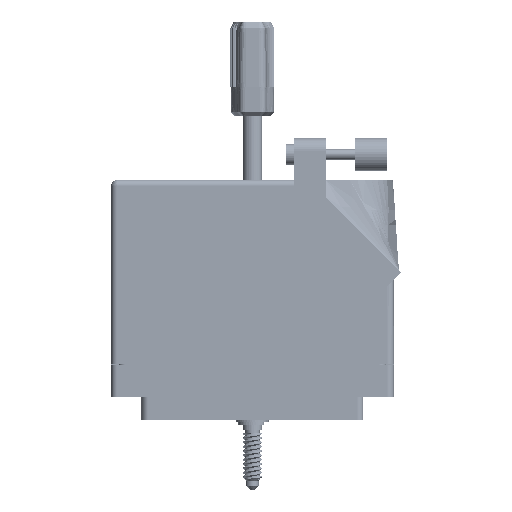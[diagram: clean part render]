
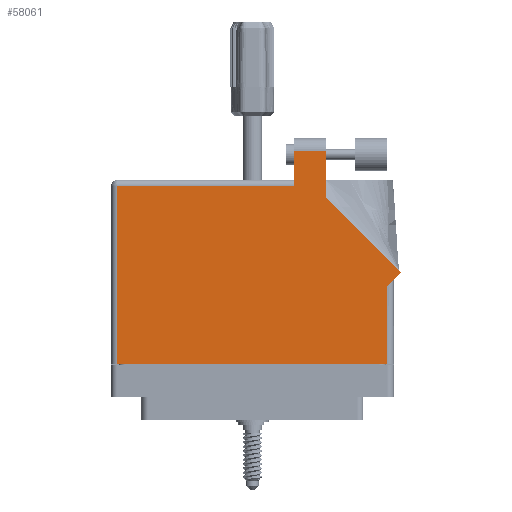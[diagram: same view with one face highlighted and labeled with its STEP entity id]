
A CAD part, front view. The second image highlights one B-rep face of the part: STEP entity #58061.
In plain terms, the highlighted face is planar.
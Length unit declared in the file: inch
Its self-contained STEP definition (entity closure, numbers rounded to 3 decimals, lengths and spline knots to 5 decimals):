
#2322 = VERTEX_POINT ( 'NONE', #53508 ) ;
#4715 = LINE ( 'NONE', #34771, #56115 ) ;
#6312 = DIRECTION ( 'NONE',  ( 0., -1., 0. ) ) ;
#9422 = CARTESIAN_POINT ( 'NONE',  ( 1.297, 0.653, 0.617 ) ) ;
#10979 = VECTOR ( 'NONE', #77867, 39.37008 ) ;
#12098 = AXIS2_PLACEMENT_3D ( 'NONE', #58994, #39095, #46079 ) ;
#12374 = EDGE_CURVE ( 'NONE', #52562, #39592, #4715, .T. ) ;
#12663 = PLANE ( 'NONE',  #12098 ) ;
#14549 = VERTEX_POINT ( 'NONE', #64242 ) ;
#15652 = EDGE_LOOP ( 'NONE', ( #80241, #50006, #67165, #20343, #57111, #83037, #20977, #72256, #41765 ) ) ;
#16289 = CARTESIAN_POINT ( 'NONE',  ( -1.297, -0.1, 0.617 ) ) ;
#16480 = DIRECTION ( 'NONE',  ( 0., 1., 0. ) ) ;
#18268 = CARTESIAN_POINT ( 'NONE',  ( 0.399, 1.613, 0.617 ) ) ;
#18974 = VERTEX_POINT ( 'NONE', #31408 ) ;
#20343 = ORIENTED_EDGE ( 'NONE', *, *, #22584, .T. ) ;
#20977 = ORIENTED_EDGE ( 'NONE', *, *, #83880, .T. ) ;
#22584 = EDGE_CURVE ( 'NONE', #84639, #2322, #63732, .T. ) ;
#23260 = LINE ( 'NONE', #41619, #76675 ) ;
#24016 = CARTESIAN_POINT ( 'NONE',  ( 0.399, 1.675, 0.617 ) ) ;
#26100 = CARTESIAN_POINT ( 'NONE',  ( -1.297, -0.1, 0.617 ) ) ;
#29074 = DIRECTION ( 'NONE',  ( 0., 1., 0. ) ) ;
#30995 = CARTESIAN_POINT ( 'NONE',  ( 1.359, 0.715, 0.617 ) ) ;
#31408 = CARTESIAN_POINT ( 'NONE',  ( 0.399, 1.95, 0.617 ) ) ;
#33461 = EDGE_CURVE ( 'NONE', #49750, #46860, #74212, .T. ) ;
#33723 = EDGE_CURVE ( 'NONE', #14549, #49750, #42667, .T. ) ;
#34771 = CARTESIAN_POINT ( 'NONE',  ( -1.359, -0.1, 0.617 ) ) ;
#36642 = VERTEX_POINT ( 'NONE', #9422 ) ;
#38726 = CARTESIAN_POINT ( 'NONE',  ( 1.42971, 0.78571, 0.617 ) ) ;
#39095 = DIRECTION ( 'NONE',  ( 0., 0., -1. ) ) ;
#39592 = VERTEX_POINT ( 'NONE', #65286 ) ;
#40361 = FACE_OUTER_BOUND ( 'NONE', #15652, .T. ) ;
#41442 = LINE ( 'NONE', #30995, #10979 ) ;
#41619 = CARTESIAN_POINT ( 'NONE',  ( 0.399, 1.95, 0.617 ) ) ;
#41765 = ORIENTED_EDGE ( 'NONE', *, *, #33723, .T. ) ;
#42085 = LINE ( 'NONE', #24016, #53551 ) ;
#42655 = VECTOR ( 'NONE', #29074, 39.37008 ) ;
#42667 = LINE ( 'NONE', #38726, #66748 ) ;
#46079 = DIRECTION ( 'NONE',  ( -1., 0., 0. ) ) ;
#46646 = EDGE_CURVE ( 'NONE', #2322, #52562, #70155, .T. ) ;
#46860 = VERTEX_POINT ( 'NONE', #82495 ) ;
#48883 = CARTESIAN_POINT ( 'NONE',  ( 0.706, 1.50942, 0.617 ) ) ;
#49091 = DIRECTION ( 'NONE',  ( 1., 0., 0. ) ) ;
#49750 = VERTEX_POINT ( 'NONE', #48883 ) ;
#50006 = ORIENTED_EDGE ( 'NONE', *, *, #50678, .T. ) ;
#50678 = EDGE_CURVE ( 'NONE', #46860, #18974, #23260, .T. ) ;
#52351 = VECTOR ( 'NONE', #6312, 39.37008 ) ;
#52562 = VERTEX_POINT ( 'NONE', #16289 ) ;
#53508 = CARTESIAN_POINT ( 'NONE',  ( -1.297, 1.613, 0.617 ) ) ;
#53551 = VECTOR ( 'NONE', #85095, 39.37008 ) ;
#56115 = VECTOR ( 'NONE', #49091, 39.37008 ) ;
#57111 = ORIENTED_EDGE ( 'NONE', *, *, #46646, .T. ) ;
#58061 = ADVANCED_FACE ( 'NONE', ( #40361 ), #12663, .F. ) ;
#58994 = CARTESIAN_POINT ( 'NONE',  ( -1.359, 1.675, 0.617 ) ) ;
#61193 = DIRECTION ( 'NONE',  ( -1., 0., 0. ) ) ;
#63732 = LINE ( 'NONE', #72027, #79472 ) ;
#64242 = CARTESIAN_POINT ( 'NONE',  ( 1.42971, 0.78571, 0.617 ) ) ;
#64453 = DIRECTION ( 'NONE',  ( -1., 0., 0. ) ) ;
#65286 = CARTESIAN_POINT ( 'NONE',  ( 1.297, -0.1, 0.617 ) ) ;
#65343 = DIRECTION ( 'NONE',  ( -0.707, 0.707, 0. ) ) ;
#66748 = VECTOR ( 'NONE', #65343, 39.37008 ) ;
#67165 = ORIENTED_EDGE ( 'NONE', *, *, #70257, .T. ) ;
#69723 = CARTESIAN_POINT ( 'NONE',  ( 1.297, 0.715, 0.617 ) ) ;
#70155 = LINE ( 'NONE', #26100, #52351 ) ;
#70257 = EDGE_CURVE ( 'NONE', #18974, #84639, #42085, .T. ) ;
#70341 = CARTESIAN_POINT ( 'NONE',  ( 0.706, 1.50942, 0.617 ) ) ;
#71959 = LINE ( 'NONE', #69723, #42655 ) ;
#72027 = CARTESIAN_POINT ( 'NONE',  ( -1.359, 1.613, 0.617 ) ) ;
#72256 = ORIENTED_EDGE ( 'NONE', *, *, #74407, .T. ) ;
#74212 = LINE ( 'NONE', #70341, #85699 ) ;
#74407 = EDGE_CURVE ( 'NONE', #36642, #14549, #41442, .T. ) ;
#76675 = VECTOR ( 'NONE', #61193, 39.37008 ) ;
#77867 = DIRECTION ( 'NONE',  ( 0.707, 0.707, 0. ) ) ;
#79472 = VECTOR ( 'NONE', #64453, 39.37008 ) ;
#80241 = ORIENTED_EDGE ( 'NONE', *, *, #33461, .T. ) ;
#82495 = CARTESIAN_POINT ( 'NONE',  ( 0.706, 1.95, 0.617 ) ) ;
#83037 = ORIENTED_EDGE ( 'NONE', *, *, #12374, .T. ) ;
#83880 = EDGE_CURVE ( 'NONE', #39592, #36642, #71959, .T. ) ;
#84639 = VERTEX_POINT ( 'NONE', #18268 ) ;
#85095 = DIRECTION ( 'NONE',  ( 0., -1., 0. ) ) ;
#85699 = VECTOR ( 'NONE', #16480, 39.37008 ) ;
